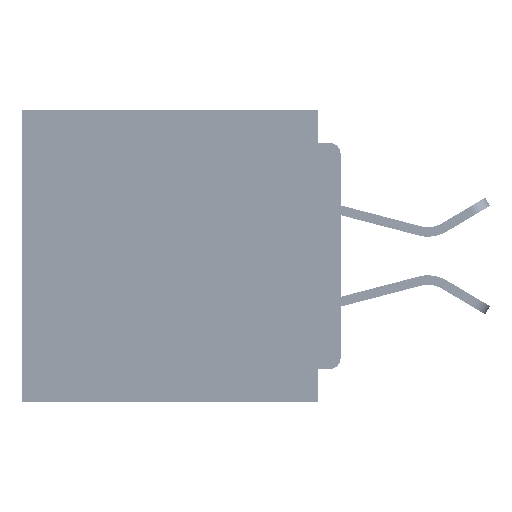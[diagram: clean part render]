
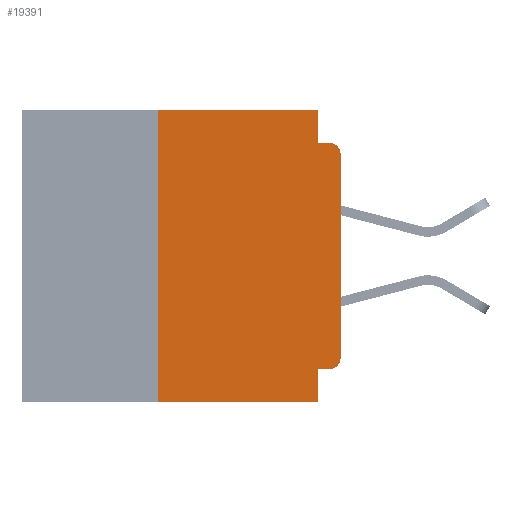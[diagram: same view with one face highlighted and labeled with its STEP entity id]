
A CAD part, left-side view. The second image highlights one B-rep face of the part: STEP entity #19391.
In plain terms, the highlighted planar face has unit normal (-1, 0, 0).
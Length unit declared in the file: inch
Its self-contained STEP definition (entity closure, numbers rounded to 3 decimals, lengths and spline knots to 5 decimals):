
#142 = VERTEX_POINT ( 'NONE', #26041 ) ;
#379 = EDGE_CURVE ( 'NONE', #6925, #6610, #8042, .T. ) ;
#1482 = AXIS2_PLACEMENT_3D ( 'NONE', #42167, #16767, #46418 ) ;
#2422 = VERTEX_POINT ( 'NONE', #31792 ) ;
#2641 = CARTESIAN_POINT ( 'NONE',  ( 0., 0.031, 0. ) ) ;
#2652 = VERTEX_POINT ( 'NONE', #12387 ) ;
#3191 = EDGE_CURVE ( 'NONE', #23090, #2422, #14455, .T. ) ;
#3585 = CARTESIAN_POINT ( 'NONE',  ( 0., 0.437, 0. ) ) ;
#4310 = ORIENTED_EDGE ( 'NONE', *, *, #47702, .T. ) ;
#4460 = CARTESIAN_POINT ( 'NONE',  ( 0., 0.031, -0.355 ) ) ;
#5262 = CARTESIAN_POINT ( 'NONE',  ( 0., 0., -0.355 ) ) ;
#5392 = DIRECTION ( 'NONE',  ( 1., 0., 0. ) ) ;
#6610 = VERTEX_POINT ( 'NONE', #43032 ) ;
#6925 = VERTEX_POINT ( 'NONE', #15362 ) ;
#7605 = EDGE_CURVE ( 'NONE', #42585, #26707, #51261, .T. ) ;
#7887 = DIRECTION ( 'NONE',  ( 0., -1., 0. ) ) ;
#8042 = LINE ( 'NONE', #53685, #40539 ) ;
#8132 = ORIENTED_EDGE ( 'NONE', *, *, #11046, .F. ) ;
#8522 = CARTESIAN_POINT ( 'NONE',  ( 0., 0.437, -0.4 ) ) ;
#9223 = VECTOR ( 'NONE', #24146, 39.37008 ) ;
#10955 = ORIENTED_EDGE ( 'NONE', *, *, #3191, .F. ) ;
#11046 = EDGE_CURVE ( 'NONE', #52729, #6925, #20306, .T. ) ;
#12014 = VECTOR ( 'NONE', #38189, 39.37008 ) ;
#12026 = EDGE_LOOP ( 'NONE', ( #18269, #4310, #13069, #8132, #39473, #53440, #42543, #10955, #19480, #28383 ) ) ;
#12387 = CARTESIAN_POINT ( 'NONE',  ( 0., 0.015, -0.355 ) ) ;
#12683 = DIRECTION ( 'NONE',  ( 0., -1., 0. ) ) ;
#13069 = ORIENTED_EDGE ( 'NONE', *, *, #379, .F. ) ;
#14455 = LINE ( 'NONE', #41915, #46927 ) ;
#14494 = VECTOR ( 'NONE', #34995, 39.37008 ) ;
#14738 = CIRCLE ( 'NONE', #24770, 0.015 ) ;
#14836 = EDGE_CURVE ( 'NONE', #142, #45490, #54304, .T. ) ;
#15170 = EDGE_CURVE ( 'NONE', #2652, #23090, #46970, .T. ) ;
#15362 = CARTESIAN_POINT ( 'NONE',  ( 0., 0.031, -0.045 ) ) ;
#16148 = CARTESIAN_POINT ( 'NONE',  ( 0., 0.015, -0.34 ) ) ;
#16767 = DIRECTION ( 'NONE',  ( -1., 0., 0. ) ) ;
#18269 = ORIENTED_EDGE ( 'NONE', *, *, #14836, .T. ) ;
#19391 = ADVANCED_FACE ( 'NONE', ( #42596 ), #26668, .F. ) ;
#19399 = LINE ( 'NONE', #3585, #40585 ) ;
#19480 = ORIENTED_EDGE ( 'NONE', *, *, #15170, .F. ) ;
#19721 = CARTESIAN_POINT ( 'NONE',  ( 0., 0.031, 0. ) ) ;
#20306 = LINE ( 'NONE', #19721, #41504 ) ;
#20451 = DIRECTION ( 'NONE',  ( 0., 0., -1. ) ) ;
#23090 = VERTEX_POINT ( 'NONE', #4460 ) ;
#23306 = LINE ( 'NONE', #8522, #12014 ) ;
#24005 = DIRECTION ( 'NONE',  ( 0., 0., -1. ) ) ;
#24146 = DIRECTION ( 'NONE',  ( 0., 0., 1. ) ) ;
#24770 = AXIS2_PLACEMENT_3D ( 'NONE', #16148, #45810, #20451 ) ;
#26041 = CARTESIAN_POINT ( 'NONE',  ( 0., 0., -0.34 ) ) ;
#26668 = PLANE ( 'NONE',  #29705 ) ;
#26707 = VERTEX_POINT ( 'NONE', #40815 ) ;
#27443 = VECTOR ( 'NONE', #38114, 39.37008 ) ;
#28383 = ORIENTED_EDGE ( 'NONE', *, *, #38803, .T. ) ;
#29231 = EDGE_CURVE ( 'NONE', #26707, #52729, #19399, .T. ) ;
#29705 = AXIS2_PLACEMENT_3D ( 'NONE', #30907, #5392, #35123 ) ;
#30907 = CARTESIAN_POINT ( 'NONE',  ( 0., 0.437, 0. ) ) ;
#31792 = CARTESIAN_POINT ( 'NONE',  ( 0., 0.031, -0.4 ) ) ;
#33084 = CARTESIAN_POINT ( 'NONE',  ( 0., 0., -0.06 ) ) ;
#33883 = CARTESIAN_POINT ( 'NONE',  ( 0., 0.25, -0.4 ) ) ;
#34995 = DIRECTION ( 'NONE',  ( 0., 1., 0. ) ) ;
#35123 = DIRECTION ( 'NONE',  ( 0., 0., -1. ) ) ;
#36137 = CARTESIAN_POINT ( 'NONE',  ( 0., 0.25, -0.4 ) ) ;
#37787 = CIRCLE ( 'NONE', #1482, 0.015 ) ;
#38114 = DIRECTION ( 'NONE',  ( 0., 0., 1. ) ) ;
#38189 = DIRECTION ( 'NONE',  ( 0., -1., 0. ) ) ;
#38803 = EDGE_CURVE ( 'NONE', #2652, #142, #14738, .T. ) ;
#39473 = ORIENTED_EDGE ( 'NONE', *, *, #29231, .F. ) ;
#40416 = EDGE_CURVE ( 'NONE', #42585, #2422, #23306, .T. ) ;
#40539 = VECTOR ( 'NONE', #12683, 39.37008 ) ;
#40585 = VECTOR ( 'NONE', #7887, 39.37008 ) ;
#40815 = CARTESIAN_POINT ( 'NONE',  ( 0., 0.25, 0. ) ) ;
#41504 = VECTOR ( 'NONE', #24005, 39.37008 ) ;
#41727 = DIRECTION ( 'NONE',  ( 0., 0., -1. ) ) ;
#41915 = CARTESIAN_POINT ( 'NONE',  ( 0., 0.031, -0.4 ) ) ;
#42167 = CARTESIAN_POINT ( 'NONE',  ( 0., 0.015, -0.06 ) ) ;
#42543 = ORIENTED_EDGE ( 'NONE', *, *, #40416, .T. ) ;
#42585 = VERTEX_POINT ( 'NONE', #36137 ) ;
#42596 = FACE_OUTER_BOUND ( 'NONE', #12026, .T. ) ;
#43032 = CARTESIAN_POINT ( 'NONE',  ( 0., 0.015, -0.045 ) ) ;
#45490 = VERTEX_POINT ( 'NONE', #33084 ) ;
#45810 = DIRECTION ( 'NONE',  ( -1., 0., 0. ) ) ;
#46418 = DIRECTION ( 'NONE',  ( 0., 0., -1. ) ) ;
#46927 = VECTOR ( 'NONE', #41727, 39.37008 ) ;
#46970 = LINE ( 'NONE', #5262, #14494 ) ;
#47702 = EDGE_CURVE ( 'NONE', #45490, #6610, #37787, .T. ) ;
#49473 = CARTESIAN_POINT ( 'NONE',  ( 0., 0., 0. ) ) ;
#51261 = LINE ( 'NONE', #33883, #27443 ) ;
#52729 = VERTEX_POINT ( 'NONE', #2641 ) ;
#53440 = ORIENTED_EDGE ( 'NONE', *, *, #7605, .F. ) ;
#53685 = CARTESIAN_POINT ( 'NONE',  ( 0., 0., -0.045 ) ) ;
#54304 = LINE ( 'NONE', #49473, #9223 ) ;
